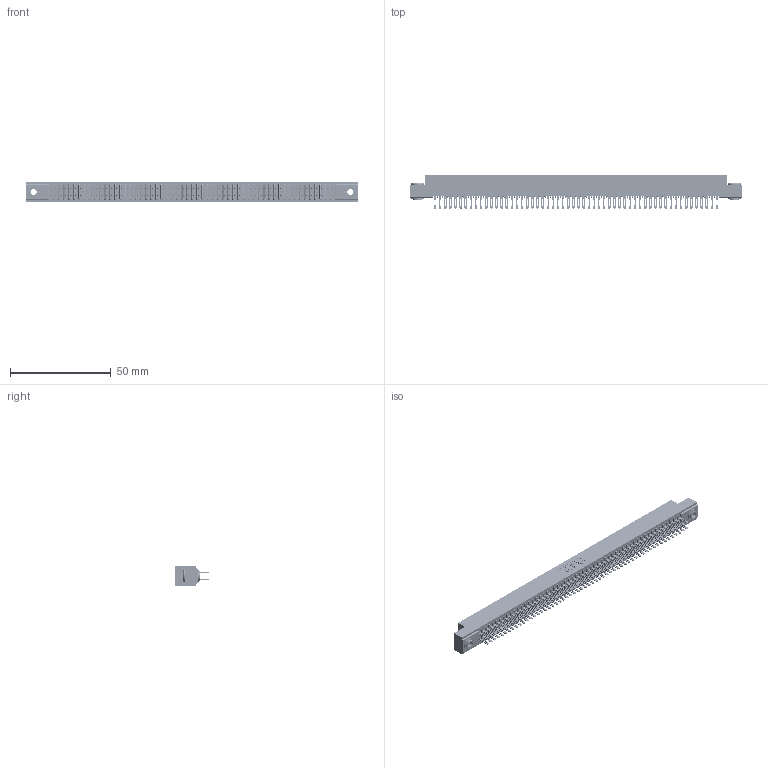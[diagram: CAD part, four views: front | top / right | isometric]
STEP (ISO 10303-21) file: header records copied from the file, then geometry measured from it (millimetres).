
FILE_DESCRIPTION (( 'STEP AP203' ), '1' );
FILE_NAME ('341-112-500-203.STEP', '2018-08-08T12:58:03', ( '' ), ( '' ), 'SwSTEP 2.0', 'SolidWorks 2016', '' );
FILE_SCHEMA (( 'CONFIG_CONTROL_DESIGN' ));
Length unit declared in the file: inch
Products named in the file (4): 341 Part_.156 (3.96) Dia Mounting Holes; 341-292-001_341-292-100; 345-250-002_345-250-002-102; 341-112-500-203
Assembly tree (115 placements, depth 2):
  341-112-500-203
    341 Part_.156 (3.96) Dia Mounting Holes
    341-292-001_341-292-100  x112
    345-250-002_345-250-002-102  x2
Bounding box: 164.47 x 16.69 x 10.16 mm (x, y, z)
Volume: 12303.2 mm3; surface area: 23459.8 mm2
Topology: 115 solids, 115 shells, 7560 faces, 21876 edges, 14166 vertices
Faces by surface type: plane 4348, cylinder 2980, sphere 114, torus 110, cone 8
Entity records: 66980 total; most frequent: CARTESIAN_POINT 11113, ORIENTED_EDGE 11036, DIRECTION 10794, EDGE_CURVE 5518, LINE 4460, VECTOR 4460, VERTEX_POINT 3486, AXIS2_PLACEMENT_3D 3167
